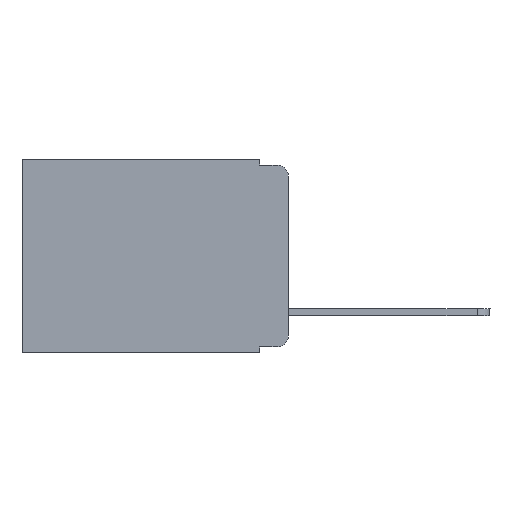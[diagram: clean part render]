
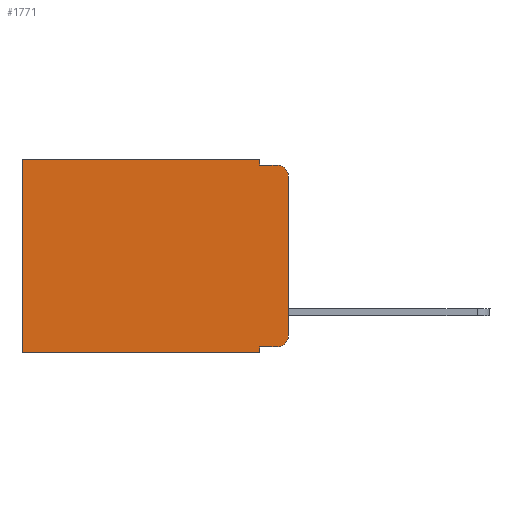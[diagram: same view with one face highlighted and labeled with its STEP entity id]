
A CAD part, left-side view. The second image highlights one B-rep face of the part: STEP entity #1771.
In plain terms, the highlighted planar face has unit normal (-1, 0, 0).
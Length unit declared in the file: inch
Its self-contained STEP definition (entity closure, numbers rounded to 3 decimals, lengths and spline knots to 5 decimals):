
#296 = DIRECTION ( 'NONE',  ( 0., 0., -1. ) ) ;
#397 = DIRECTION ( 'NONE',  ( 1., 0., 0. ) ) ;
#576 = EDGE_CURVE ( 'NONE', #11386, #13863, #12455, .T. ) ;
#587 = ORIENTED_EDGE ( 'NONE', *, *, #19113, .F. ) ;
#631 = LINE ( 'NONE', #6682, #1541 ) ;
#1541 = VECTOR ( 'NONE', #12714, 39.37008 ) ;
#1577 = LINE ( 'NONE', #4446, #18498 ) ;
#1770 = EDGE_CURVE ( 'NONE', #10954, #17777, #14890, .T. ) ;
#1771 = ADVANCED_FACE ( 'NONE', ( #9973 ), #17131, .F. ) ;
#1845 = ORIENTED_EDGE ( 'NONE', *, *, #5109, .T. ) ;
#2062 = CIRCLE ( 'NONE', #10305, 0.02 ) ;
#2082 = AXIS2_PLACEMENT_3D ( 'NONE', #10818, #397, #12484 ) ;
#2511 = ORIENTED_EDGE ( 'NONE', *, *, #10808, .T. ) ;
#2742 = CARTESIAN_POINT ( 'NONE',  ( 0.298, 0.051, -0.333 ) ) ;
#2784 = DIRECTION ( 'NONE',  ( 0., 1., 0. ) ) ;
#2949 = DIRECTION ( 'NONE',  ( 0., -1., 0. ) ) ;
#3110 = VECTOR ( 'NONE', #15036, 39.37008 ) ;
#3131 = EDGE_LOOP ( 'NONE', ( #8979, #2511, #17801, #4579, #15149, #4319, #587, #7808, #1845, #8911 ) ) ;
#3173 = CARTESIAN_POINT ( 'NONE',  ( 0.298, 0.051, -0.333 ) ) ;
#3434 = EDGE_CURVE ( 'NONE', #7426, #8615, #18098, .T. ) ;
#3946 = DIRECTION ( 'NONE',  ( -1., 0., 0. ) ) ;
#4026 = CARTESIAN_POINT ( 'NONE',  ( 0.298, 0.02, -0.01 ) ) ;
#4319 = ORIENTED_EDGE ( 'NONE', *, *, #5293, .T. ) ;
#4349 = CARTESIAN_POINT ( 'NONE',  ( 0.298, 0.02, -0.313 ) ) ;
#4446 = CARTESIAN_POINT ( 'NONE',  ( 0.298, 0.051, -0.01 ) ) ;
#4547 = DIRECTION ( 'NONE',  ( 0., 0., -1. ) ) ;
#4579 = ORIENTED_EDGE ( 'NONE', *, *, #15076, .F. ) ;
#4683 = VECTOR ( 'NONE', #4547, 39.37008 ) ;
#5109 = EDGE_CURVE ( 'NONE', #7426, #11386, #7617, .T. ) ;
#5293 = EDGE_CURVE ( 'NONE', #17777, #13521, #18261, .T. ) ;
#6199 = VECTOR ( 'NONE', #2784, 39.37008 ) ;
#6335 = VERTEX_POINT ( 'NONE', #4026 ) ;
#6682 = CARTESIAN_POINT ( 'NONE',  ( 0.298, 0., -0.343 ) ) ;
#7223 = DIRECTION ( 'NONE',  ( 0., 0., -1. ) ) ;
#7426 = VERTEX_POINT ( 'NONE', #3173 ) ;
#7617 = LINE ( 'NONE', #2742, #3110 ) ;
#7808 = ORIENTED_EDGE ( 'NONE', *, *, #3434, .F. ) ;
#7832 = LINE ( 'NONE', #13880, #17887 ) ;
#8615 = VERTEX_POINT ( 'NONE', #14898 ) ;
#8813 = VECTOR ( 'NONE', #16802, 39.37008 ) ;
#8863 = DIRECTION ( 'NONE',  ( 0., 0., -1. ) ) ;
#8911 = ORIENTED_EDGE ( 'NONE', *, *, #576, .T. ) ;
#8979 = ORIENTED_EDGE ( 'NONE', *, *, #11473, .F. ) ;
#9158 = CARTESIAN_POINT ( 'NONE',  ( 0.298, 0.051, 0. ) ) ;
#9323 = CARTESIAN_POINT ( 'NONE',  ( 0.298, 0.02, -0.333 ) ) ;
#9713 = CARTESIAN_POINT ( 'NONE',  ( 0.298, 0.473, -0.343 ) ) ;
#9972 = VECTOR ( 'NONE', #18497, 39.37008 ) ;
#9973 = FACE_OUTER_BOUND ( 'NONE', #3131, .T. ) ;
#9990 = EDGE_CURVE ( 'NONE', #15061, #6335, #1577, .T. ) ;
#10253 = CARTESIAN_POINT ( 'NONE',  ( 0.298, 0.473, 0. ) ) ;
#10305 = AXIS2_PLACEMENT_3D ( 'NONE', #13419, #12022, #8863 ) ;
#10699 = CARTESIAN_POINT ( 'NONE',  ( 0.298, 0.051, 0. ) ) ;
#10769 = CARTESIAN_POINT ( 'NONE',  ( 0.298, 0.473, 0. ) ) ;
#10808 = EDGE_CURVE ( 'NONE', #13888, #6335, #2062, .T. ) ;
#10818 = CARTESIAN_POINT ( 'NONE',  ( 0.298, 0., 0. ) ) ;
#10954 = VERTEX_POINT ( 'NONE', #9158 ) ;
#10989 = CARTESIAN_POINT ( 'NONE',  ( 0.298, 0., -0.313 ) ) ;
#11386 = VERTEX_POINT ( 'NONE', #9323 ) ;
#11473 = EDGE_CURVE ( 'NONE', #13888, #13863, #15747, .T. ) ;
#12022 = DIRECTION ( 'NONE',  ( -1., 0., 0. ) ) ;
#12455 = CIRCLE ( 'NONE', #12774, 0.02 ) ;
#12484 = DIRECTION ( 'NONE',  ( 0., 0., -1. ) ) ;
#12714 = DIRECTION ( 'NONE',  ( 0., 1., 0. ) ) ;
#12774 = AXIS2_PLACEMENT_3D ( 'NONE', #4349, #3946, #7223 ) ;
#13419 = CARTESIAN_POINT ( 'NONE',  ( 0.298, 0.02, -0.03 ) ) ;
#13521 = VERTEX_POINT ( 'NONE', #9713 ) ;
#13863 = VERTEX_POINT ( 'NONE', #10989 ) ;
#13877 = CARTESIAN_POINT ( 'NONE',  ( 0.298, 0., -0.03 ) ) ;
#13880 = CARTESIAN_POINT ( 'NONE',  ( 0.298, 0.051, 0. ) ) ;
#13888 = VERTEX_POINT ( 'NONE', #13877 ) ;
#14185 = CARTESIAN_POINT ( 'NONE',  ( 0.298, 0., 0. ) ) ;
#14890 = LINE ( 'NONE', #16348, #6199 ) ;
#14898 = CARTESIAN_POINT ( 'NONE',  ( 0.298, 0.051, -0.343 ) ) ;
#15036 = DIRECTION ( 'NONE',  ( 0., -1., 0. ) ) ;
#15061 = VERTEX_POINT ( 'NONE', #16832 ) ;
#15076 = EDGE_CURVE ( 'NONE', #10954, #15061, #7832, .T. ) ;
#15149 = ORIENTED_EDGE ( 'NONE', *, *, #1770, .T. ) ;
#15747 = LINE ( 'NONE', #14185, #9972 ) ;
#16348 = CARTESIAN_POINT ( 'NONE',  ( 0.298, 0., 0. ) ) ;
#16802 = DIRECTION ( 'NONE',  ( 0., 0., -1. ) ) ;
#16832 = CARTESIAN_POINT ( 'NONE',  ( 0.298, 0.051, -0.01 ) ) ;
#17131 = PLANE ( 'NONE',  #2082 ) ;
#17777 = VERTEX_POINT ( 'NONE', #10253 ) ;
#17801 = ORIENTED_EDGE ( 'NONE', *, *, #9990, .F. ) ;
#17887 = VECTOR ( 'NONE', #296, 39.37008 ) ;
#18098 = LINE ( 'NONE', #10699, #4683 ) ;
#18261 = LINE ( 'NONE', #10769, #8813 ) ;
#18497 = DIRECTION ( 'NONE',  ( 0., 0., -1. ) ) ;
#18498 = VECTOR ( 'NONE', #2949, 39.37008 ) ;
#19113 = EDGE_CURVE ( 'NONE', #8615, #13521, #631, .T. ) ;
